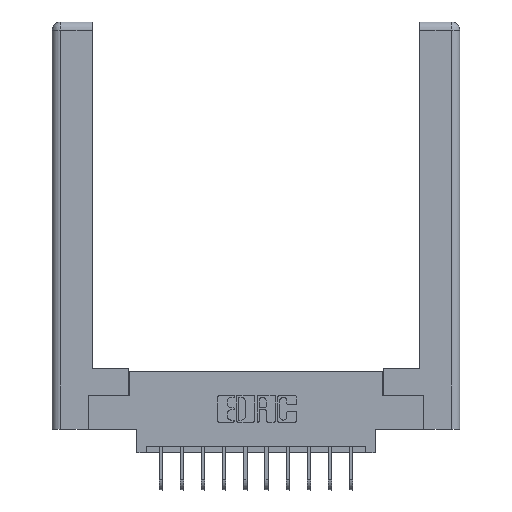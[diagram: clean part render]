
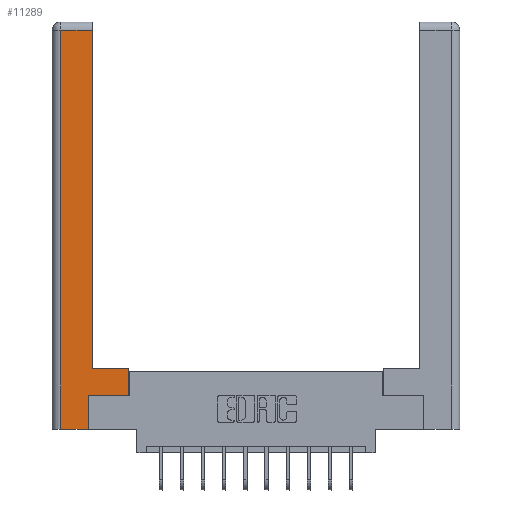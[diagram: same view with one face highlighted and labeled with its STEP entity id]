
A CAD part, top view. The second image highlights one B-rep face of the part: STEP entity #11289.
In plain terms, the highlighted planar face has unit normal (0, 0, 1).
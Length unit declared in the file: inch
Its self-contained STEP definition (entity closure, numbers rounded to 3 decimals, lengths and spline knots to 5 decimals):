
#378 = VERTEX_POINT ( 'NONE', #4255 ) ;
#402 = LINE ( 'NONE', #3805, #11416 ) ;
#602 = EDGE_CURVE ( 'NONE', #2459, #1018, #5673, .T. ) ;
#674 = VECTOR ( 'NONE', #2132, 39.37008 ) ;
#1018 = VERTEX_POINT ( 'NONE', #12574 ) ;
#1092 = ORIENTED_EDGE ( 'NONE', *, *, #2040, .T. ) ;
#1347 = CARTESIAN_POINT ( 'NONE',  ( 0.265, 0.245, 0. ) ) ;
#2040 = EDGE_CURVE ( 'NONE', #2375, #378, #4262, .T. ) ;
#2132 = DIRECTION ( 'NONE',  ( 0., -1., 0. ) ) ;
#2177 = ORIENTED_EDGE ( 'NONE', *, *, #3049, .T. ) ;
#2375 = VERTEX_POINT ( 'NONE', #11744 ) ;
#2459 = VERTEX_POINT ( 'NONE', #10959 ) ;
#2603 = LINE ( 'NONE', #14398, #674 ) ;
#2632 = LINE ( 'NONE', #7340, #2823 ) ;
#2823 = VECTOR ( 'NONE', #14118, 39.37008 ) ;
#2976 = CARTESIAN_POINT ( 'NONE',  ( 0.0615, 2.94, 0. ) ) ;
#3008 = VERTEX_POINT ( 'NONE', #4588 ) ;
#3049 = EDGE_CURVE ( 'NONE', #1018, #11038, #2632, .T. ) ;
#3398 = VECTOR ( 'NONE', #14327, 39.37008 ) ;
#3805 = CARTESIAN_POINT ( 'NONE',  ( 0.295, 3., 0. ) ) ;
#4229 = VERTEX_POINT ( 'NONE', #11840 ) ;
#4255 = CARTESIAN_POINT ( 'NONE',  ( 0.265, 0.245, 0. ) ) ;
#4262 = LINE ( 'NONE', #1347, #6495 ) ;
#4588 = CARTESIAN_POINT ( 'NONE',  ( 0.0615, 2.94, 0. ) ) ;
#4875 = AXIS2_PLACEMENT_3D ( 'NONE', #8204, #6921, #13742 ) ;
#5093 = DIRECTION ( 'NONE',  ( 1., 0., 0. ) ) ;
#5426 = ORIENTED_EDGE ( 'NONE', *, *, #11767, .T. ) ;
#5673 = LINE ( 'NONE', #8675, #10933 ) ;
#5756 = DIRECTION ( 'NONE',  ( 0., 1., 0. ) ) ;
#6078 = FACE_OUTER_BOUND ( 'NONE', #11973, .T. ) ;
#6495 = VECTOR ( 'NONE', #5756, 39.37008 ) ;
#6786 = ORIENTED_EDGE ( 'NONE', *, *, #9610, .T. ) ;
#6921 = DIRECTION ( 'NONE',  ( 0., 0., -1. ) ) ;
#7070 = PLANE ( 'NONE',  #4875 ) ;
#7149 = DIRECTION ( 'NONE',  ( 0., 1., 0. ) ) ;
#7340 = CARTESIAN_POINT ( 'NONE',  ( 0.295, 0.45, 0. ) ) ;
#7354 = DIRECTION ( 'NONE',  ( 0., 1., 0. ) ) ;
#7388 = LINE ( 'NONE', #13319, #3398 ) ;
#8073 = LINE ( 'NONE', #2976, #9490 ) ;
#8204 = CARTESIAN_POINT ( 'NONE',  ( 0., 0., 0. ) ) ;
#8487 = DIRECTION ( 'NONE',  ( -1., 0., 0. ) ) ;
#8575 = EDGE_CURVE ( 'NONE', #11038, #4229, #402, .T. ) ;
#8675 = CARTESIAN_POINT ( 'NONE',  ( 0.565, 0.45, 0. ) ) ;
#8764 = EDGE_CURVE ( 'NONE', #4229, #3008, #8073, .T. ) ;
#9413 = ORIENTED_EDGE ( 'NONE', *, *, #11023, .T. ) ;
#9490 = VECTOR ( 'NONE', #8487, 39.37008 ) ;
#9610 = EDGE_CURVE ( 'NONE', #378, #2459, #11557, .T. ) ;
#9618 = ORIENTED_EDGE ( 'NONE', *, *, #8764, .T. ) ;
#10127 = ORIENTED_EDGE ( 'NONE', *, *, #8575, .T. ) ;
#10191 = ORIENTED_EDGE ( 'NONE', *, *, #602, .T. ) ;
#10933 = VECTOR ( 'NONE', #7354, 39.37008 ) ;
#10959 = CARTESIAN_POINT ( 'NONE',  ( 0.565, 0.245, 0. ) ) ;
#11023 = EDGE_CURVE ( 'NONE', #3008, #11376, #2603, .T. ) ;
#11038 = VERTEX_POINT ( 'NONE', #13286 ) ;
#11289 = ADVANCED_FACE ( 'NONE', ( #6078 ), #7070, .F. ) ;
#11376 = VERTEX_POINT ( 'NONE', #13702 ) ;
#11416 = VECTOR ( 'NONE', #7149, 39.37008 ) ;
#11557 = LINE ( 'NONE', #12953, #14144 ) ;
#11744 = CARTESIAN_POINT ( 'NONE',  ( 0.265, 0., 0. ) ) ;
#11767 = EDGE_CURVE ( 'NONE', #11376, #2375, #7388, .T. ) ;
#11840 = CARTESIAN_POINT ( 'NONE',  ( 0.295, 2.94, 0. ) ) ;
#11973 = EDGE_LOOP ( 'NONE', ( #10127, #9618, #9413, #5426, #1092, #6786, #10191, #2177 ) ) ;
#12574 = CARTESIAN_POINT ( 'NONE',  ( 0.565, 0.45, 0. ) ) ;
#12953 = CARTESIAN_POINT ( 'NONE',  ( 0.565, 0.245, 0. ) ) ;
#13286 = CARTESIAN_POINT ( 'NONE',  ( 0.295, 0.45, 0. ) ) ;
#13319 = CARTESIAN_POINT ( 'NONE',  ( 0.265, 0., 0. ) ) ;
#13702 = CARTESIAN_POINT ( 'NONE',  ( 0.0615, 0., 0. ) ) ;
#13742 = DIRECTION ( 'NONE',  ( -1., 0., 0. ) ) ;
#14118 = DIRECTION ( 'NONE',  ( -1., 0., 0. ) ) ;
#14144 = VECTOR ( 'NONE', #5093, 39.37008 ) ;
#14327 = DIRECTION ( 'NONE',  ( 1., 0., 0. ) ) ;
#14398 = CARTESIAN_POINT ( 'NONE',  ( 0.0615, 0., 0. ) ) ;
